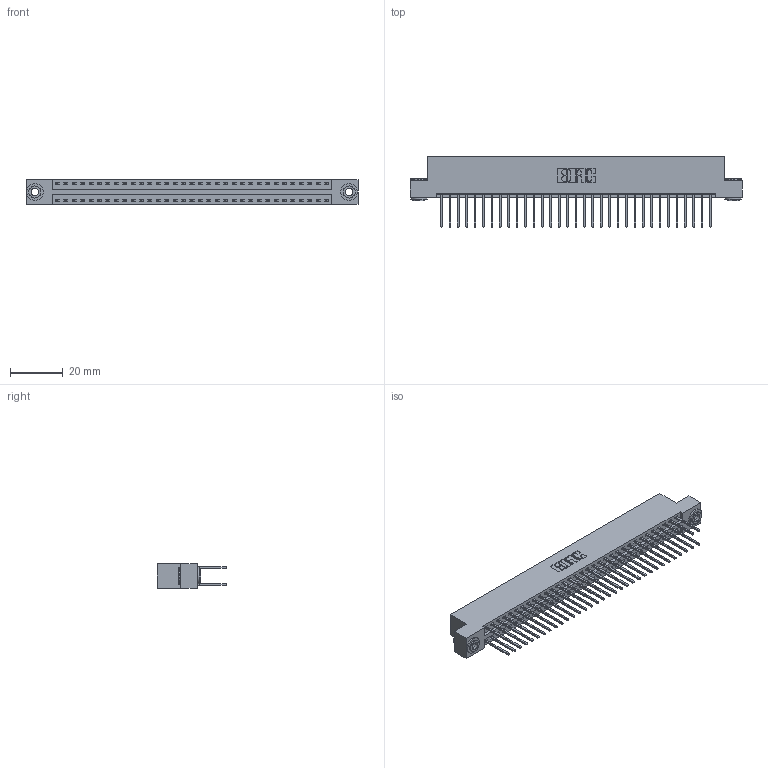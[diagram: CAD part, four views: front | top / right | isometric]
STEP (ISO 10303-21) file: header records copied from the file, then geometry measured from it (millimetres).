
FILE_DESCRIPTION (( 'STEP AP203' ), '1' );
FILE_NAME ('346-066-522-203.STEP', '2022-05-24T16:56:23', ( '' ), ( '' ), 'SwSTEP 2.0', 'SolidWorks 2020', '' );
FILE_SCHEMA (( 'CONFIG_CONTROL_DESIGN' ));
Length unit declared in the file: inch
Products named in the file (4): 346-066-522-203; 345-250-002_345-250-002-102; 346 Part_Flush Mounting Lugs - 0.156 Dia-TH; 345-292-001_345-293-122
Assembly tree (69 placements, depth 2):
  346-066-522-203
    346 Part_Flush Mounting Lugs - 0.156 Dia-TH
    345-292-001_345-293-122  x66
    345-250-002_345-250-002-102  x2
Bounding box: 125.35 x 26.42 x 9.4 mm (x, y, z)
Volume: 12323.6 mm3; surface area: 17830.8 mm2
Topology: 69 solids, 69 shells, 3606 faces, 10671 edges, 7022 vertices
Faces by surface type: plane 2410, cylinder 1188, cone 8
Entity records: 23832 total; most frequent: CARTESIAN_POINT 3921, ORIENTED_EDGE 3846, DIRECTION 3537, EDGE_CURVE 1923, LINE 1635, VECTOR 1635, VERTEX_POINT 1278, AXIS2_PLACEMENT_3D 951
